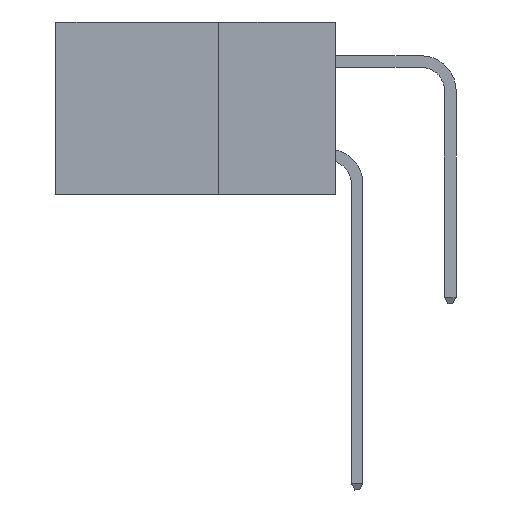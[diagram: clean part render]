
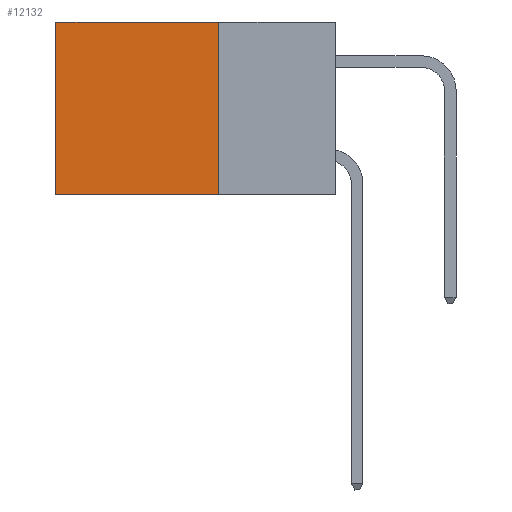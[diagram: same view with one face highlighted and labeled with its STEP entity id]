
A CAD part, left-side view. The second image highlights one B-rep face of the part: STEP entity #12132.
In plain terms, the highlighted planar face has unit normal (-1, 0, 0).
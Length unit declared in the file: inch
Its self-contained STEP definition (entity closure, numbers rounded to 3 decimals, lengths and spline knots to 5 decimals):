
#609 = CARTESIAN_POINT ( 'NONE',  ( 0.2875, 0.25, 0. ) ) ;
#1876 = ORIENTED_EDGE ( 'NONE', *, *, #8835, .T. ) ;
#1906 = VERTEX_POINT ( 'NONE', #2615 ) ;
#2615 = CARTESIAN_POINT ( 'NONE',  ( 0.2875, 0.25, 0. ) ) ;
#3028 = ORIENTED_EDGE ( 'NONE', *, *, #10162, .F. ) ;
#3411 = ORIENTED_EDGE ( 'NONE', *, *, #11833, .F. ) ;
#3688 = VECTOR ( 'NONE', #10309, 39.37008 ) ;
#4986 = DIRECTION ( 'NONE',  ( 0., 0., -1. ) ) ;
#5109 = VERTEX_POINT ( 'NONE', #14238 ) ;
#5359 = VECTOR ( 'NONE', #13365, 39.37008 ) ;
#5480 = VERTEX_POINT ( 'NONE', #12432 ) ;
#5506 = DIRECTION ( 'NONE',  ( 1., 0., 0. ) ) ;
#5545 = AXIS2_PLACEMENT_3D ( 'NONE', #609, #5506, #13562 ) ;
#5685 = VECTOR ( 'NONE', #5736, 39.37008 ) ;
#5736 = DIRECTION ( 'NONE',  ( 0., 1., 0. ) ) ;
#6294 = CARTESIAN_POINT ( 'NONE',  ( 0.2875, 0.6, -0.37 ) ) ;
#6434 = CARTESIAN_POINT ( 'NONE',  ( 0.2875, 0.6, 0. ) ) ;
#6893 = CARTESIAN_POINT ( 'NONE',  ( 0.2875, 0.25, -0.37 ) ) ;
#6909 = ORIENTED_EDGE ( 'NONE', *, *, #14055, .T. ) ;
#7122 = VERTEX_POINT ( 'NONE', #6294 ) ;
#7191 = LINE ( 'NONE', #9210, #3688 ) ;
#7276 = VECTOR ( 'NONE', #4986, 39.37008 ) ;
#8835 = EDGE_CURVE ( 'NONE', #5109, #7122, #11469, .T. ) ;
#9210 = CARTESIAN_POINT ( 'NONE',  ( 0.2875, 0.25, 0. ) ) ;
#9411 = FACE_OUTER_BOUND ( 'NONE', #12234, .T. ) ;
#10162 = EDGE_CURVE ( 'NONE', #5480, #7122, #11796, .T. ) ;
#10309 = DIRECTION ( 'NONE',  ( 0., 1., 0. ) ) ;
#10650 = LINE ( 'NONE', #10723, #7276 ) ;
#10723 = CARTESIAN_POINT ( 'NONE',  ( 0.2875, 0.25, 0. ) ) ;
#11469 = LINE ( 'NONE', #6434, #5359 ) ;
#11796 = LINE ( 'NONE', #6893, #5685 ) ;
#11833 = EDGE_CURVE ( 'NONE', #1906, #5480, #10650, .T. ) ;
#12132 = ADVANCED_FACE ( 'NONE', ( #9411 ), #12413, .F. ) ;
#12234 = EDGE_LOOP ( 'NONE', ( #1876, #3028, #3411, #6909 ) ) ;
#12413 = PLANE ( 'NONE',  #5545 ) ;
#12432 = CARTESIAN_POINT ( 'NONE',  ( 0.2875, 0.25, -0.37 ) ) ;
#13365 = DIRECTION ( 'NONE',  ( 0., 0., -1. ) ) ;
#13562 = DIRECTION ( 'NONE',  ( 0., 0., -1. ) ) ;
#14055 = EDGE_CURVE ( 'NONE', #1906, #5109, #7191, .T. ) ;
#14238 = CARTESIAN_POINT ( 'NONE',  ( 0.2875, 0.6, 0. ) ) ;
